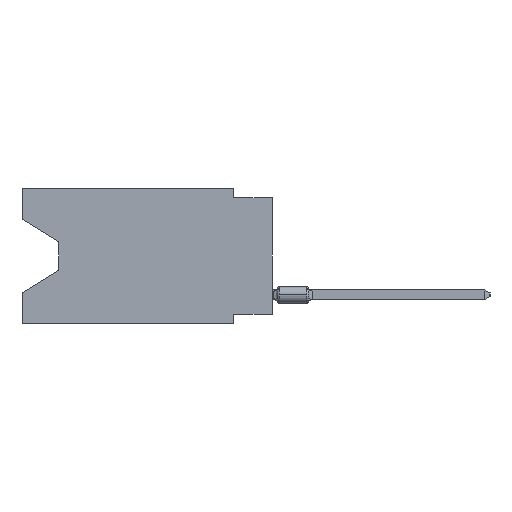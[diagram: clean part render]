
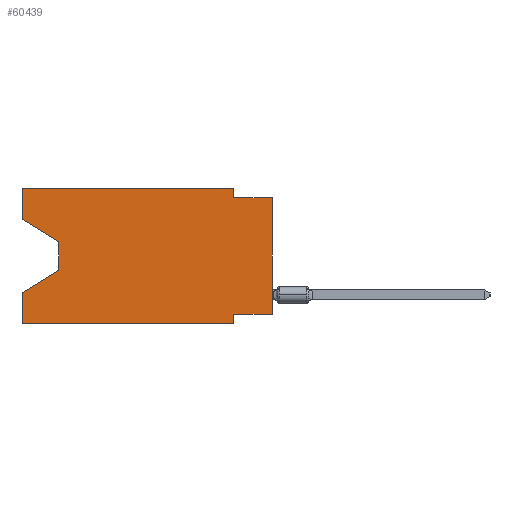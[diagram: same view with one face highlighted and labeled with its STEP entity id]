
A CAD part, left-side view. The second image highlights one B-rep face of the part: STEP entity #60439.
In plain terms, the highlighted planar face has unit normal (-1, 0, 0).
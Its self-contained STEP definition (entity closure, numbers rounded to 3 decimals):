
#360 = DIRECTION ( 'NONE',  ( 0., 0., 1. ) ) ;
#1392 = VECTOR ( 'NONE', #360, 1000. ) ;
#1849 = LINE ( 'NONE', #12872, #17854 ) ;
#2659 = ORIENTED_EDGE ( 'NONE', *, *, #66005, .F. ) ;
#2918 = VECTOR ( 'NONE', #54547, 1000. ) ;
#4053 = VECTOR ( 'NONE', #63593, 1000. ) ;
#4288 = CARTESIAN_POINT ( 'NONE',  ( 0., 13.97, -5.385 ) ) ;
#5139 = LINE ( 'NONE', #25527, #59072 ) ;
#5375 = CARTESIAN_POINT ( 'NONE',  ( 0., 16.383, 0. ) ) ;
#5872 = LINE ( 'NONE', #30610, #32704 ) ;
#7441 = VECTOR ( 'NONE', #38893, 1000. ) ;
#7847 = LINE ( 'NONE', #48608, #7441 ) ;
#8471 = EDGE_CURVE ( 'NONE', #34135, #65596, #5872, .T. ) ;
#9675 = VERTEX_POINT ( 'NONE', #19295 ) ;
#10737 = LINE ( 'NONE', #15425, #49132 ) ;
#11193 = LINE ( 'NONE', #21545, #36476 ) ;
#11378 = LINE ( 'NONE', #38030, #12620 ) ;
#11871 = VERTEX_POINT ( 'NONE', #46906 ) ;
#12177 = CARTESIAN_POINT ( 'NONE',  ( 0., 2.54, -0.635 ) ) ;
#12620 = VECTOR ( 'NONE', #63127, 1000. ) ;
#12872 = CARTESIAN_POINT ( 'NONE',  ( 0., 16.383, 0. ) ) ;
#13432 = CARTESIAN_POINT ( 'NONE',  ( 0., 0., -0.635 ) ) ;
#14421 = CARTESIAN_POINT ( 'NONE',  ( 0., 0., -8.255 ) ) ;
#14772 = CARTESIAN_POINT ( 'NONE',  ( 0., 16.383, -2.038 ) ) ;
#14950 = VECTOR ( 'NONE', #19467, 1000. ) ;
#15425 = CARTESIAN_POINT ( 'NONE',  ( 0., 13.97, -3.505 ) ) ;
#16740 = FACE_OUTER_BOUND ( 'NONE', #50730, .T. ) ;
#17156 = ORIENTED_EDGE ( 'NONE', *, *, #54474, .F. ) ;
#17669 = CARTESIAN_POINT ( 'NONE',  ( 0., 16.383, -2.038 ) ) ;
#17854 = VECTOR ( 'NONE', #22228, 1000. ) ;
#17976 = ORIENTED_EDGE ( 'NONE', *, *, #47416, .F. ) ;
#18476 = CARTESIAN_POINT ( 'NONE',  ( 0., 16.383, 0. ) ) ;
#19295 = CARTESIAN_POINT ( 'NONE',  ( 0., 2.54, 0. ) ) ;
#19467 = DIRECTION ( 'NONE',  ( 0., -0.855, -0.519 ) ) ;
#19551 = VERTEX_POINT ( 'NONE', #14421 ) ;
#21448 = ORIENTED_EDGE ( 'NONE', *, *, #35809, .F. ) ;
#21545 = CARTESIAN_POINT ( 'NONE',  ( 0., 0., -0.635 ) ) ;
#21580 = DIRECTION ( 'NONE',  ( 0., 0., -1. ) ) ;
#22228 = DIRECTION ( 'NONE',  ( 0., 0., 1. ) ) ;
#22709 = EDGE_CURVE ( 'NONE', #19551, #57681, #27529, .T. ) ;
#24215 = LINE ( 'NONE', #34241, #59556 ) ;
#25527 = CARTESIAN_POINT ( 'NONE',  ( 0., 16.383, -8.89 ) ) ;
#26283 = CARTESIAN_POINT ( 'NONE',  ( 0., 13.97, -3.505 ) ) ;
#27098 = CARTESIAN_POINT ( 'NONE',  ( 0., 16.383, 0. ) ) ;
#27262 = ORIENTED_EDGE ( 'NONE', *, *, #51704, .T. ) ;
#27529 = LINE ( 'NONE', #43218, #4053 ) ;
#30610 = CARTESIAN_POINT ( 'NONE',  ( 0., 2.54, -8.89 ) ) ;
#31445 = EDGE_CURVE ( 'NONE', #43086, #11871, #57147, .T. ) ;
#32704 = VECTOR ( 'NONE', #21580, 1000. ) ;
#32729 = PLANE ( 'NONE',  #33093 ) ;
#33093 = AXIS2_PLACEMENT_3D ( 'NONE', #27098, #62817, #42426 ) ;
#33152 = ORIENTED_EDGE ( 'NONE', *, *, #36097, .F. ) ;
#34135 = VERTEX_POINT ( 'NONE', #59718 ) ;
#34241 = CARTESIAN_POINT ( 'NONE',  ( 0., 13.97, -5.385 ) ) ;
#35809 = EDGE_CURVE ( 'NONE', #11871, #9675, #58878, .T. ) ;
#36097 = EDGE_CURVE ( 'NONE', #63100, #45039, #1849, .T. ) ;
#36476 = VECTOR ( 'NONE', #62304, 1000. ) ;
#37276 = CARTESIAN_POINT ( 'NONE',  ( 0., 16.383, -8.89 ) ) ;
#37337 = VERTEX_POINT ( 'NONE', #4288 ) ;
#38030 = CARTESIAN_POINT ( 'NONE',  ( 0., 2.54, 0. ) ) ;
#38477 = VERTEX_POINT ( 'NONE', #26283 ) ;
#38664 = EDGE_CURVE ( 'NONE', #37337, #45039, #24215, .T. ) ;
#38893 = DIRECTION ( 'NONE',  ( 0., 1., 0. ) ) ;
#40147 = LINE ( 'NONE', #14772, #14950 ) ;
#40554 = DIRECTION ( 'NONE',  ( 0., -1., 0. ) ) ;
#42426 = DIRECTION ( 'NONE',  ( 0., 0., -1. ) ) ;
#43086 = VERTEX_POINT ( 'NONE', #17669 ) ;
#43218 = CARTESIAN_POINT ( 'NONE',  ( 0., 0., 0. ) ) ;
#43980 = VERTEX_POINT ( 'NONE', #12177 ) ;
#44798 = ORIENTED_EDGE ( 'NONE', *, *, #22709, .T. ) ;
#45039 = VERTEX_POINT ( 'NONE', #61954 ) ;
#46906 = CARTESIAN_POINT ( 'NONE',  ( 0., 16.383, 0. ) ) ;
#46973 = ORIENTED_EDGE ( 'NONE', *, *, #8471, .F. ) ;
#47416 = EDGE_CURVE ( 'NONE', #9675, #43980, #11378, .T. ) ;
#48608 = CARTESIAN_POINT ( 'NONE',  ( 0., 0., -8.255 ) ) ;
#49132 = VECTOR ( 'NONE', #55169, 1000. ) ;
#49288 = DIRECTION ( 'NONE',  ( 0., 0.855, -0.519 ) ) ;
#50730 = EDGE_LOOP ( 'NONE', ( #27262, #62700, #57479, #33152, #59159, #46973, #2659, #44798, #17156, #17976, #21448, #61094 ) ) ;
#51704 = EDGE_CURVE ( 'NONE', #43086, #38477, #40147, .T. ) ;
#54474 = EDGE_CURVE ( 'NONE', #43980, #57681, #11193, .T. ) ;
#54547 = DIRECTION ( 'NONE',  ( 0., -1., 0. ) ) ;
#55169 = DIRECTION ( 'NONE',  ( 0., 0., -1. ) ) ;
#56599 = EDGE_CURVE ( 'NONE', #63100, #65596, #5139, .T. ) ;
#57147 = LINE ( 'NONE', #5375, #1392 ) ;
#57479 = ORIENTED_EDGE ( 'NONE', *, *, #38664, .T. ) ;
#57681 = VERTEX_POINT ( 'NONE', #13432 ) ;
#58878 = LINE ( 'NONE', #18476, #2918 ) ;
#59072 = VECTOR ( 'NONE', #40554, 1000. ) ;
#59159 = ORIENTED_EDGE ( 'NONE', *, *, #56599, .T. ) ;
#59362 = CARTESIAN_POINT ( 'NONE',  ( 0., 2.54, -8.89 ) ) ;
#59556 = VECTOR ( 'NONE', #49288, 1000. ) ;
#59718 = CARTESIAN_POINT ( 'NONE',  ( 0., 2.54, -8.255 ) ) ;
#60306 = EDGE_CURVE ( 'NONE', #38477, #37337, #10737, .T. ) ;
#60439 = ADVANCED_FACE ( 'NONE', ( #16740 ), #32729, .F. ) ;
#61094 = ORIENTED_EDGE ( 'NONE', *, *, #31445, .F. ) ;
#61954 = CARTESIAN_POINT ( 'NONE',  ( 0., 16.383, -6.852 ) ) ;
#62304 = DIRECTION ( 'NONE',  ( 0., -1., 0. ) ) ;
#62700 = ORIENTED_EDGE ( 'NONE', *, *, #60306, .T. ) ;
#62817 = DIRECTION ( 'NONE',  ( 1., 0., 0. ) ) ;
#63100 = VERTEX_POINT ( 'NONE', #37276 ) ;
#63127 = DIRECTION ( 'NONE',  ( 0., 0., -1. ) ) ;
#63593 = DIRECTION ( 'NONE',  ( 0., 0., 1. ) ) ;
#65596 = VERTEX_POINT ( 'NONE', #59362 ) ;
#66005 = EDGE_CURVE ( 'NONE', #19551, #34135, #7847, .T. ) ;
